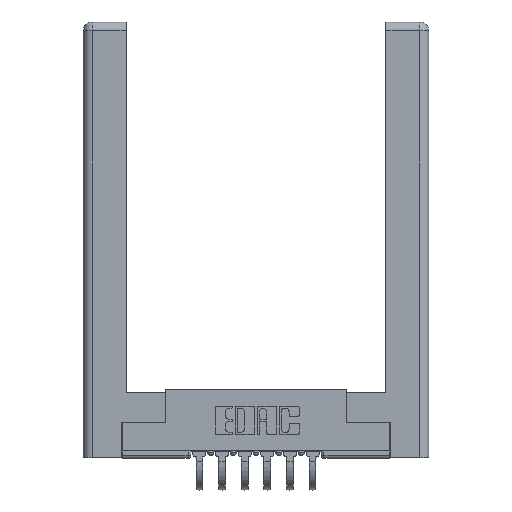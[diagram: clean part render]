
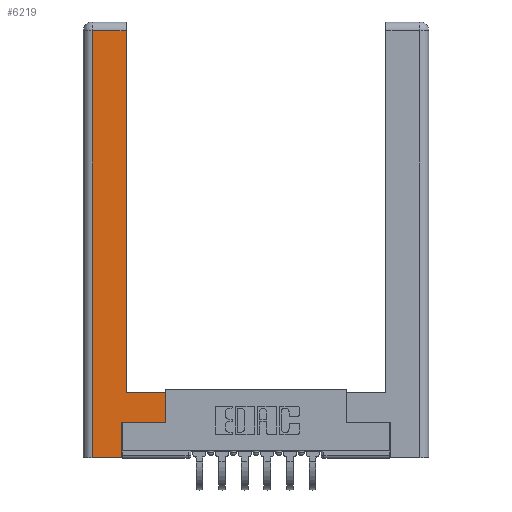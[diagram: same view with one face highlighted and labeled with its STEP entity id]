
A CAD part, top view. The second image highlights one B-rep face of the part: STEP entity #6219.
In plain terms, the highlighted planar face has unit normal (0, 0, 1).
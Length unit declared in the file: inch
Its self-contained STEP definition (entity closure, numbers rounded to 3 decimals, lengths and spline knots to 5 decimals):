
#92 = VERTEX_POINT ( 'NONE', #5626 ) ;
#544 = CARTESIAN_POINT ( 'NONE',  ( 0.0615, 2.94, 0. ) ) ;
#547 = CARTESIAN_POINT ( 'NONE',  ( 0.295, 0.45, 0. ) ) ;
#606 = LINE ( 'NONE', #9238, #1964 ) ;
#684 = EDGE_CURVE ( 'NONE', #1407, #11494, #9951, .T. ) ;
#880 = CARTESIAN_POINT ( 'NONE',  ( 0.0615, 0., 0. ) ) ;
#937 = VECTOR ( 'NONE', #7067, 39.37008 ) ;
#1218 = ORIENTED_EDGE ( 'NONE', *, *, #2674, .T. ) ;
#1257 = EDGE_CURVE ( 'NONE', #92, #6293, #11549, .T. ) ;
#1407 = VERTEX_POINT ( 'NONE', #9497 ) ;
#1464 = LINE ( 'NONE', #9818, #12368 ) ;
#1634 = VECTOR ( 'NONE', #13191, 39.37008 ) ;
#1638 = DIRECTION ( 'NONE',  ( 0., 0., -1. ) ) ;
#1806 = CARTESIAN_POINT ( 'NONE',  ( 0.265, 0., 0. ) ) ;
#1829 = VECTOR ( 'NONE', #2840, 39.37008 ) ;
#1956 = VERTEX_POINT ( 'NONE', #547 ) ;
#1964 = VECTOR ( 'NONE', #9169, 39.37008 ) ;
#2674 = EDGE_CURVE ( 'NONE', #11494, #4015, #3333, .T. ) ;
#2689 = FACE_OUTER_BOUND ( 'NONE', #5563, .T. ) ;
#2840 = DIRECTION ( 'NONE',  ( 0., 1., 0. ) ) ;
#3333 = LINE ( 'NONE', #7398, #13315 ) ;
#3531 = LINE ( 'NONE', #12026, #13594 ) ;
#3764 = CARTESIAN_POINT ( 'NONE',  ( 0.265, 0.245, 0. ) ) ;
#3991 = EDGE_CURVE ( 'NONE', #6293, #1956, #12416, .T. ) ;
#4015 = VERTEX_POINT ( 'NONE', #880 ) ;
#4019 = VERTEX_POINT ( 'NONE', #1806 ) ;
#4121 = LINE ( 'NONE', #8595, #9797 ) ;
#4475 = ORIENTED_EDGE ( 'NONE', *, *, #11626, .T. ) ;
#4561 = DIRECTION ( 'NONE',  ( 1., 0., 0. ) ) ;
#4897 = ORIENTED_EDGE ( 'NONE', *, *, #11020, .T. ) ;
#5204 = CARTESIAN_POINT ( 'NONE',  ( 0.565, 0.45, 0. ) ) ;
#5563 = EDGE_LOOP ( 'NONE', ( #8824, #11216, #1218, #4475, #4897, #7165, #11477, #10623 ) ) ;
#5626 = CARTESIAN_POINT ( 'NONE',  ( 0.565, 0.245, 0. ) ) ;
#6073 = CARTESIAN_POINT ( 'NONE',  ( 0.565, 0.45, 0. ) ) ;
#6175 = DIRECTION ( 'NONE',  ( -1., 0., 0. ) ) ;
#6219 = ADVANCED_FACE ( 'NONE', ( #2689 ), #6967, .F. ) ;
#6293 = VERTEX_POINT ( 'NONE', #5204 ) ;
#6473 = EDGE_CURVE ( 'NONE', #12802, #92, #1464, .T. ) ;
#6625 = DIRECTION ( 'NONE',  ( 0., -1., 0. ) ) ;
#6967 = PLANE ( 'NONE',  #9212 ) ;
#7067 = DIRECTION ( 'NONE',  ( -1., 0., 0. ) ) ;
#7165 = ORIENTED_EDGE ( 'NONE', *, *, #6473, .T. ) ;
#7398 = CARTESIAN_POINT ( 'NONE',  ( 0.0615, 0., 0. ) ) ;
#8595 = CARTESIAN_POINT ( 'NONE',  ( 0.265, 0.245, 0. ) ) ;
#8824 = ORIENTED_EDGE ( 'NONE', *, *, #10788, .T. ) ;
#9169 = DIRECTION ( 'NONE',  ( 0., 1., 0. ) ) ;
#9212 = AXIS2_PLACEMENT_3D ( 'NONE', #11255, #1638, #6175 ) ;
#9238 = CARTESIAN_POINT ( 'NONE',  ( 0.295, 3., 0. ) ) ;
#9497 = CARTESIAN_POINT ( 'NONE',  ( 0.295, 2.94, 0. ) ) ;
#9770 = DIRECTION ( 'NONE',  ( 1., 0., 0. ) ) ;
#9797 = VECTOR ( 'NONE', #12893, 39.37008 ) ;
#9818 = CARTESIAN_POINT ( 'NONE',  ( 0.565, 0.245, 0. ) ) ;
#9914 = CARTESIAN_POINT ( 'NONE',  ( 0.0615, 2.94, 0. ) ) ;
#9951 = LINE ( 'NONE', #544, #1634 ) ;
#10623 = ORIENTED_EDGE ( 'NONE', *, *, #3991, .T. ) ;
#10788 = EDGE_CURVE ( 'NONE', #1956, #1407, #606, .T. ) ;
#11020 = EDGE_CURVE ( 'NONE', #4019, #12802, #4121, .T. ) ;
#11216 = ORIENTED_EDGE ( 'NONE', *, *, #684, .T. ) ;
#11255 = CARTESIAN_POINT ( 'NONE',  ( 0., 0., 0. ) ) ;
#11290 = CARTESIAN_POINT ( 'NONE',  ( 0.295, 0.45, 0. ) ) ;
#11477 = ORIENTED_EDGE ( 'NONE', *, *, #1257, .T. ) ;
#11494 = VERTEX_POINT ( 'NONE', #9914 ) ;
#11549 = LINE ( 'NONE', #6073, #1829 ) ;
#11626 = EDGE_CURVE ( 'NONE', #4015, #4019, #3531, .T. ) ;
#12026 = CARTESIAN_POINT ( 'NONE',  ( 0.265, 0., 0. ) ) ;
#12368 = VECTOR ( 'NONE', #4561, 39.37008 ) ;
#12416 = LINE ( 'NONE', #11290, #937 ) ;
#12802 = VERTEX_POINT ( 'NONE', #3764 ) ;
#12893 = DIRECTION ( 'NONE',  ( 0., 1., 0. ) ) ;
#13191 = DIRECTION ( 'NONE',  ( -1., 0., 0. ) ) ;
#13315 = VECTOR ( 'NONE', #6625, 39.37008 ) ;
#13594 = VECTOR ( 'NONE', #9770, 39.37008 ) ;
